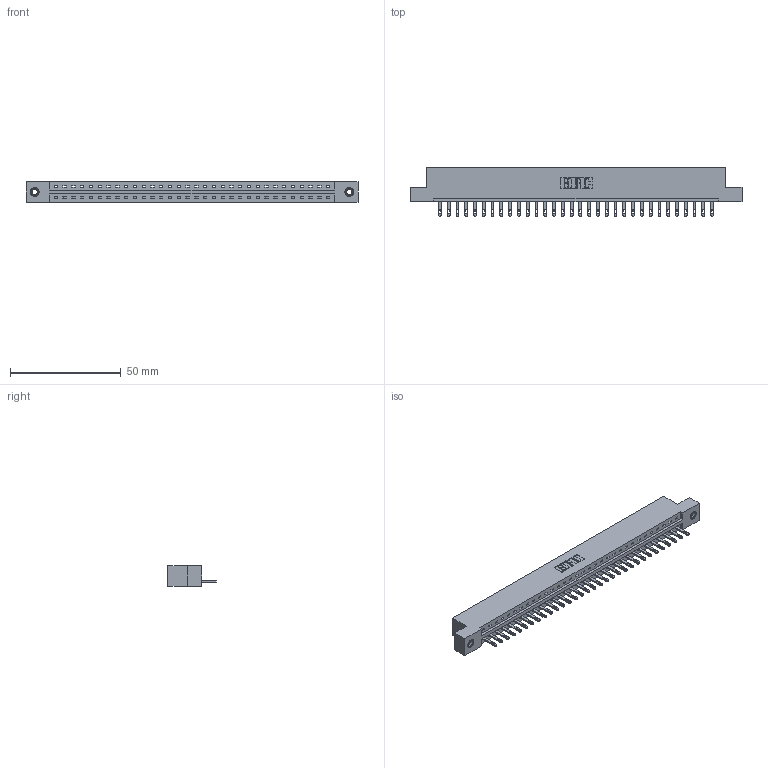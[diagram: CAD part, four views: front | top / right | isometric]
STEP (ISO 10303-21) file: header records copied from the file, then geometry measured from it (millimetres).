
FILE_DESCRIPTION (( 'STEP AP203' ), '1' );
FILE_NAME ('337-032-500-107.STEP', '2019-10-01T02:13:26', ( '' ), ( '' ), 'SwSTEP 2.0', 'SolidWorks 2016', '' );
FILE_SCHEMA (( 'CONFIG_CONTROL_DESIGN' ));
Length unit declared in the file: inch
Products named in the file (4): 345-250-001_345-250-005-103; 345-292-001_345-293-100; 337-032-500-107; 337 Part_Flush Mounting Lugs - 0.156 Dia-TI
Assembly tree (35 placements, depth 2):
  337-032-500-107
    337 Part_Flush Mounting Lugs - 0.156 Dia-TI
    345-292-001_345-293-100  x32
    345-250-001_345-250-005-103  x2
Bounding box: 149.81 x 21.85 x 9.4 mm (x, y, z)
Volume: 15451.3 mm3; surface area: 16026.9 mm2
Topology: 35 solids, 35 shells, 2030 faces, 6207 edges, 4130 vertices
Faces by surface type: plane 1382, cylinder 632, cone 12, torus 4
Entity records: 26196 total; most frequent: CARTESIAN_POINT 4541, ORIENTED_EDGE 4502, DIRECTION 3877, EDGE_CURVE 2251, LINE 2099, VECTOR 2099, VERTEX_POINT 1496, AXIS2_PLACEMENT_3D 889
